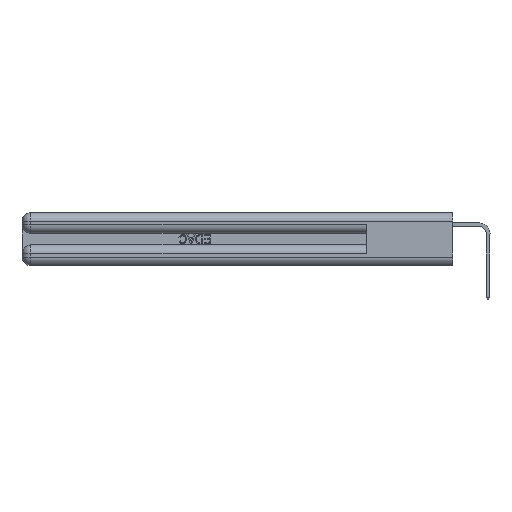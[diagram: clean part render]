
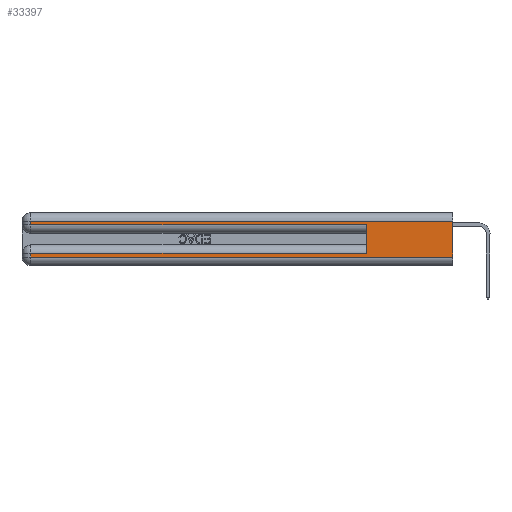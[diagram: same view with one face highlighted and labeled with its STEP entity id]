
A CAD part, left-side view. The second image highlights one B-rep face of the part: STEP entity #33397.
In plain terms, the highlighted planar face has unit normal (-1, 0, 0).
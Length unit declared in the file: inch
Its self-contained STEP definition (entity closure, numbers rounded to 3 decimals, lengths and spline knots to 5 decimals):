
#451 = EDGE_CURVE ( 'NONE', #33526, #27290, #12355, .T. ) ;
#1541 = DIRECTION ( 'NONE',  ( 0., 1., 0. ) ) ;
#2752 = LINE ( 'NONE', #10033, #34602 ) ;
#2888 = VECTOR ( 'NONE', #20856, 39.37008 ) ;
#3088 = LINE ( 'NONE', #4090, #34900 ) ;
#4090 = CARTESIAN_POINT ( 'NONE',  ( 0., 0., 0.37 ) ) ;
#5248 = EDGE_CURVE ( 'NONE', #33526, #34811, #10225, .T. ) ;
#6551 = ORIENTED_EDGE ( 'NONE', *, *, #37418, .T. ) ;
#6715 = EDGE_LOOP ( 'NONE', ( #30668, #33556, #6551, #14836, #24948, #11453, #29294, #35036 ) ) ;
#7323 = VERTEX_POINT ( 'NONE', #39227 ) ;
#7485 = CARTESIAN_POINT ( 'NONE',  ( 0., 0., 0.085 ) ) ;
#7644 = LINE ( 'NONE', #23216, #23151 ) ;
#7770 = CARTESIAN_POINT ( 'NONE',  ( 0., 0., 0.31 ) ) ;
#8961 = DIRECTION ( 'NONE',  ( 0., -1., 0. ) ) ;
#10033 = CARTESIAN_POINT ( 'NONE',  ( 0., 0., 0.285 ) ) ;
#10225 = LINE ( 'NONE', #7485, #11214 ) ;
#10485 = DIRECTION ( 'NONE',  ( 0., 0., 1. ) ) ;
#10492 = CARTESIAN_POINT ( 'NONE',  ( 0., 2.94, 0.085 ) ) ;
#11214 = VECTOR ( 'NONE', #29087, 39.37008 ) ;
#11453 = ORIENTED_EDGE ( 'NONE', *, *, #5248, .T. ) ;
#11631 = EDGE_CURVE ( 'NONE', #37670, #25324, #3088, .T. ) ;
#12355 = LINE ( 'NONE', #28922, #36820 ) ;
#13024 = CARTESIAN_POINT ( 'NONE',  ( 0., 2.94, 0.37 ) ) ;
#14836 = ORIENTED_EDGE ( 'NONE', *, *, #35406, .T. ) ;
#15481 = DIRECTION ( 'NONE',  ( 1., 0., 0. ) ) ;
#16004 = CARTESIAN_POINT ( 'NONE',  ( 0., 0.6, 0.285 ) ) ;
#16113 = DIRECTION ( 'NONE',  ( 0., 0., -1. ) ) ;
#16627 = VERTEX_POINT ( 'NONE', #31405 ) ;
#16669 = LINE ( 'NONE', #13024, #32014 ) ;
#17155 = CARTESIAN_POINT ( 'NONE',  ( 0., 0., 0.06 ) ) ;
#19039 = EDGE_CURVE ( 'NONE', #37670, #16627, #7644, .T. ) ;
#19159 = CARTESIAN_POINT ( 'NONE',  ( 0., 0.6, 0.085 ) ) ;
#20856 = DIRECTION ( 'NONE',  ( 0., 0., -1. ) ) ;
#23151 = VECTOR ( 'NONE', #1541, 39.37008 ) ;
#23216 = CARTESIAN_POINT ( 'NONE',  ( 0., 0., 0.31 ) ) ;
#24948 = ORIENTED_EDGE ( 'NONE', *, *, #451, .F. ) ;
#25324 = VERTEX_POINT ( 'NONE', #17155 ) ;
#25325 = VECTOR ( 'NONE', #8961, 39.37008 ) ;
#27290 = VERTEX_POINT ( 'NONE', #16004 ) ;
#28487 = LINE ( 'NONE', #36086, #2888 ) ;
#28801 = VERTEX_POINT ( 'NONE', #35733 ) ;
#28922 = CARTESIAN_POINT ( 'NONE',  ( 0., 0.6, 0.145 ) ) ;
#28945 = AXIS2_PLACEMENT_3D ( 'NONE', #30774, #15481, #36922 ) ;
#28986 = EDGE_CURVE ( 'NONE', #28801, #25324, #32505, .T. ) ;
#29087 = DIRECTION ( 'NONE',  ( 0., 1., 0. ) ) ;
#29294 = ORIENTED_EDGE ( 'NONE', *, *, #39787, .T. ) ;
#30515 = CARTESIAN_POINT ( 'NONE',  ( 0., 0., 0.06 ) ) ;
#30668 = ORIENTED_EDGE ( 'NONE', *, *, #11631, .F. ) ;
#30774 = CARTESIAN_POINT ( 'NONE',  ( 0., 0., 0.37 ) ) ;
#31405 = CARTESIAN_POINT ( 'NONE',  ( 0., 2.94, 0.31 ) ) ;
#31861 = DIRECTION ( 'NONE',  ( 0., 0., -1. ) ) ;
#32014 = VECTOR ( 'NONE', #16113, 39.37008 ) ;
#32505 = LINE ( 'NONE', #30515, #25325 ) ;
#33397 = ADVANCED_FACE ( 'NONE', ( #34707 ), #33855, .F. ) ;
#33526 = VERTEX_POINT ( 'NONE', #19159 ) ;
#33556 = ORIENTED_EDGE ( 'NONE', *, *, #19039, .T. ) ;
#33855 = PLANE ( 'NONE',  #28945 ) ;
#34602 = VECTOR ( 'NONE', #37724, 39.37008 ) ;
#34707 = FACE_OUTER_BOUND ( 'NONE', #6715, .T. ) ;
#34811 = VERTEX_POINT ( 'NONE', #10492 ) ;
#34900 = VECTOR ( 'NONE', #31861, 39.37008 ) ;
#35036 = ORIENTED_EDGE ( 'NONE', *, *, #28986, .T. ) ;
#35406 = EDGE_CURVE ( 'NONE', #7323, #27290, #2752, .T. ) ;
#35733 = CARTESIAN_POINT ( 'NONE',  ( 0., 2.94, 0.06 ) ) ;
#36086 = CARTESIAN_POINT ( 'NONE',  ( 0., 2.94, 0.37 ) ) ;
#36820 = VECTOR ( 'NONE', #10485, 39.37008 ) ;
#36922 = DIRECTION ( 'NONE',  ( 0., 0., -1. ) ) ;
#37418 = EDGE_CURVE ( 'NONE', #16627, #7323, #16669, .T. ) ;
#37670 = VERTEX_POINT ( 'NONE', #7770 ) ;
#37724 = DIRECTION ( 'NONE',  ( 0., -1., 0. ) ) ;
#39227 = CARTESIAN_POINT ( 'NONE',  ( 0., 2.94, 0.285 ) ) ;
#39787 = EDGE_CURVE ( 'NONE', #34811, #28801, #28487, .T. ) ;
